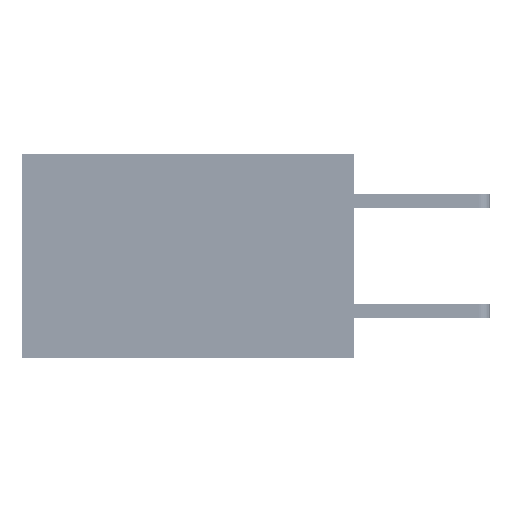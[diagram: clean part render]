
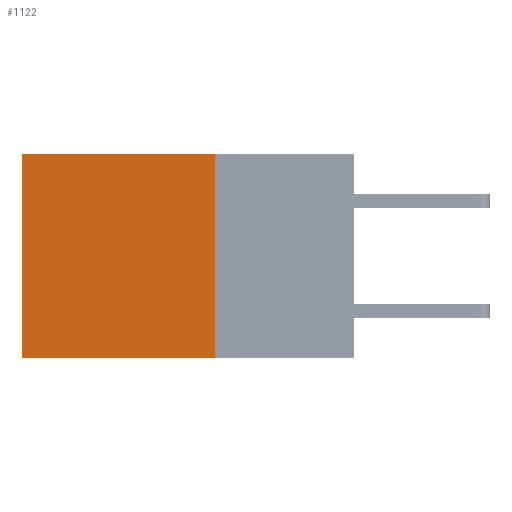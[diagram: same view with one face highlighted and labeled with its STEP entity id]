
A CAD part, left-side view. The second image highlights one B-rep face of the part: STEP entity #1122.
In plain terms, the highlighted planar face has unit normal (-1, 0, 0).
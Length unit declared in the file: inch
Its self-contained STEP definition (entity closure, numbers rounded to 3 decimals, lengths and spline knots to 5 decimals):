
#891 = LINE ( 'NONE', #15475, #19707 ) ;
#1122 = ADVANCED_FACE ( 'NONE', ( #23673 ), #33618, .F. ) ;
#3990 = EDGE_CURVE ( 'NONE', #29778, #9821, #24920, .T. ) ;
#4144 = CARTESIAN_POINT ( 'NONE',  ( 0.2875, 0.6, 0. ) ) ;
#5876 = ORIENTED_EDGE ( 'NONE', *, *, #11280, .F. ) ;
#9821 = VERTEX_POINT ( 'NONE', #24103 ) ;
#11280 = EDGE_CURVE ( 'NONE', #14027, #39499, #29670, .T. ) ;
#12884 = VECTOR ( 'NONE', #36785, 39.37008 ) ;
#14027 = VERTEX_POINT ( 'NONE', #37655 ) ;
#14050 = ORIENTED_EDGE ( 'NONE', *, *, #17092, .F. ) ;
#14901 = CARTESIAN_POINT ( 'NONE',  ( 0.2875, 0.25, 0. ) ) ;
#15068 = ORIENTED_EDGE ( 'NONE', *, *, #3990, .T. ) ;
#15475 = CARTESIAN_POINT ( 'NONE',  ( 0.2875, 0.25, -0.37 ) ) ;
#16617 = AXIS2_PLACEMENT_3D ( 'NONE', #14901, #30383, #36610 ) ;
#17092 = EDGE_CURVE ( 'NONE', #39499, #9821, #891, .T. ) ;
#17741 = CARTESIAN_POINT ( 'NONE',  ( 0.2875, 0.25, -0.37 ) ) ;
#17983 = LINE ( 'NONE', #29192, #30051 ) ;
#19707 = VECTOR ( 'NONE', #27705, 39.37008 ) ;
#23673 = FACE_OUTER_BOUND ( 'NONE', #38544, .T. ) ;
#24103 = CARTESIAN_POINT ( 'NONE',  ( 0.2875, 0.6, -0.37 ) ) ;
#24920 = LINE ( 'NONE', #30811, #12884 ) ;
#24949 = DIRECTION ( 'NONE',  ( 0., 0., -1. ) ) ;
#25237 = CARTESIAN_POINT ( 'NONE',  ( 0.2875, 0.25, 0. ) ) ;
#27705 = DIRECTION ( 'NONE',  ( 0., 1., 0. ) ) ;
#29192 = CARTESIAN_POINT ( 'NONE',  ( 0.2875, 0.25, 0. ) ) ;
#29670 = LINE ( 'NONE', #25237, #31104 ) ;
#29778 = VERTEX_POINT ( 'NONE', #4144 ) ;
#30051 = VECTOR ( 'NONE', #38503, 39.37008 ) ;
#30383 = DIRECTION ( 'NONE',  ( 1., 0., 0. ) ) ;
#30811 = CARTESIAN_POINT ( 'NONE',  ( 0.2875, 0.6, 0. ) ) ;
#31104 = VECTOR ( 'NONE', #24949, 39.37008 ) ;
#32316 = EDGE_CURVE ( 'NONE', #14027, #29778, #17983, .T. ) ;
#32538 = ORIENTED_EDGE ( 'NONE', *, *, #32316, .T. ) ;
#33618 = PLANE ( 'NONE',  #16617 ) ;
#36610 = DIRECTION ( 'NONE',  ( 0., 0., -1. ) ) ;
#36785 = DIRECTION ( 'NONE',  ( 0., 0., -1. ) ) ;
#37655 = CARTESIAN_POINT ( 'NONE',  ( 0.2875, 0.25, 0. ) ) ;
#38503 = DIRECTION ( 'NONE',  ( 0., 1., 0. ) ) ;
#38544 = EDGE_LOOP ( 'NONE', ( #15068, #14050, #5876, #32538 ) ) ;
#39499 = VERTEX_POINT ( 'NONE', #17741 ) ;
